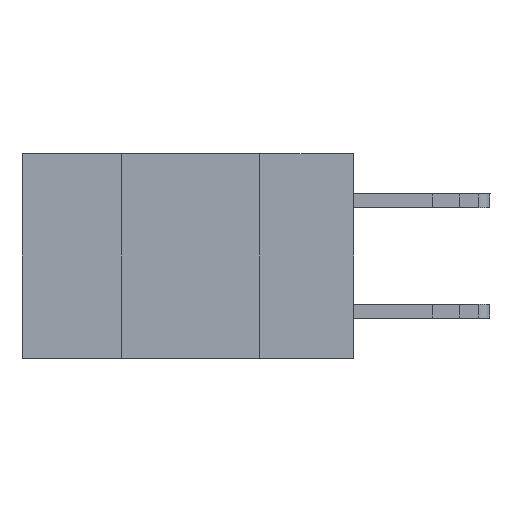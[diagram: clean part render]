
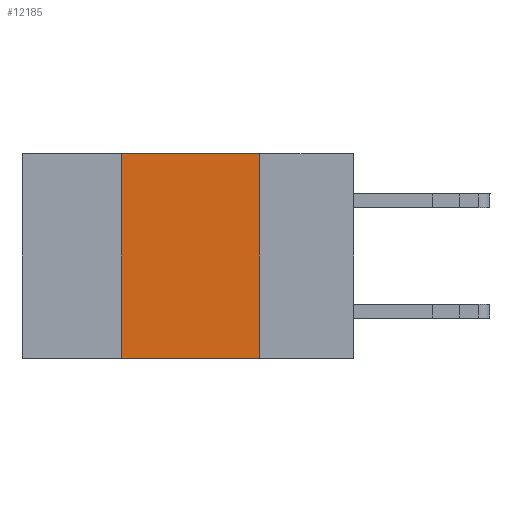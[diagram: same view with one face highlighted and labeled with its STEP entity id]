
A CAD part, left-side view. The second image highlights one B-rep face of the part: STEP entity #12185.
In plain terms, the highlighted planar face has unit normal (-1, 0, 0).
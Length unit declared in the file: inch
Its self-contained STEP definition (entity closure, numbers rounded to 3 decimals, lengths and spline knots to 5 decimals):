
#873 = LINE ( 'NONE', #2095, #14617 ) ;
#1352 = CARTESIAN_POINT ( 'NONE',  ( 0., 0.17, 0. ) ) ;
#2095 = CARTESIAN_POINT ( 'NONE',  ( 0., 0.6, 0. ) ) ;
#2777 = CARTESIAN_POINT ( 'NONE',  ( 0., 0.42, 0. ) ) ;
#4301 = VECTOR ( 'NONE', #5759, 39.37008 ) ;
#5271 = LINE ( 'NONE', #9039, #8158 ) ;
#5759 = DIRECTION ( 'NONE',  ( 0., 0., -1. ) ) ;
#6093 = EDGE_CURVE ( 'NONE', #23123, #19900, #20596, .T. ) ;
#6511 = ORIENTED_EDGE ( 'NONE', *, *, #23744, .T. ) ;
#6547 = EDGE_LOOP ( 'NONE', ( #23527, #25829, #8965, #6511 ) ) ;
#7848 = CARTESIAN_POINT ( 'NONE',  ( 0., 0.42, 0. ) ) ;
#8158 = VECTOR ( 'NONE', #12796, 39.37008 ) ;
#8478 = VERTEX_POINT ( 'NONE', #12342 ) ;
#8965 = ORIENTED_EDGE ( 'NONE', *, *, #26147, .F. ) ;
#9039 = CARTESIAN_POINT ( 'NONE',  ( 0., 0.6, -0.37 ) ) ;
#9800 = CARTESIAN_POINT ( 'NONE',  ( 0., 0.6, 0. ) ) ;
#12185 = ADVANCED_FACE ( 'NONE', ( #25959 ), #19971, .F. ) ;
#12342 = CARTESIAN_POINT ( 'NONE',  ( 0., 0.42, -0.37 ) ) ;
#12407 = LINE ( 'NONE', #7848, #18778 ) ;
#12796 = DIRECTION ( 'NONE',  ( 0., -1., 0. ) ) ;
#14537 = DIRECTION ( 'NONE',  ( 0., 0., 1. ) ) ;
#14617 = VECTOR ( 'NONE', #24723, 39.37008 ) ;
#17956 = CARTESIAN_POINT ( 'NONE',  ( 0., 0.17, 0. ) ) ;
#17996 = DIRECTION ( 'NONE',  ( 0., 0., -1. ) ) ;
#18778 = VECTOR ( 'NONE', #14537, 39.37008 ) ;
#18931 = AXIS2_PLACEMENT_3D ( 'NONE', #9800, #24025, #17996 ) ;
#19900 = VERTEX_POINT ( 'NONE', #24483 ) ;
#19971 = PLANE ( 'NONE',  #18931 ) ;
#20581 = VERTEX_POINT ( 'NONE', #2777 ) ;
#20596 = LINE ( 'NONE', #17956, #4301 ) ;
#22814 = EDGE_CURVE ( 'NONE', #20581, #23123, #873, .T. ) ;
#23123 = VERTEX_POINT ( 'NONE', #1352 ) ;
#23527 = ORIENTED_EDGE ( 'NONE', *, *, #6093, .F. ) ;
#23744 = EDGE_CURVE ( 'NONE', #8478, #19900, #5271, .T. ) ;
#24025 = DIRECTION ( 'NONE',  ( 1., 0., 0. ) ) ;
#24483 = CARTESIAN_POINT ( 'NONE',  ( 0., 0.17, -0.37 ) ) ;
#24723 = DIRECTION ( 'NONE',  ( 0., -1., 0. ) ) ;
#25829 = ORIENTED_EDGE ( 'NONE', *, *, #22814, .F. ) ;
#25959 = FACE_OUTER_BOUND ( 'NONE', #6547, .T. ) ;
#26147 = EDGE_CURVE ( 'NONE', #8478, #20581, #12407, .T. ) ;
